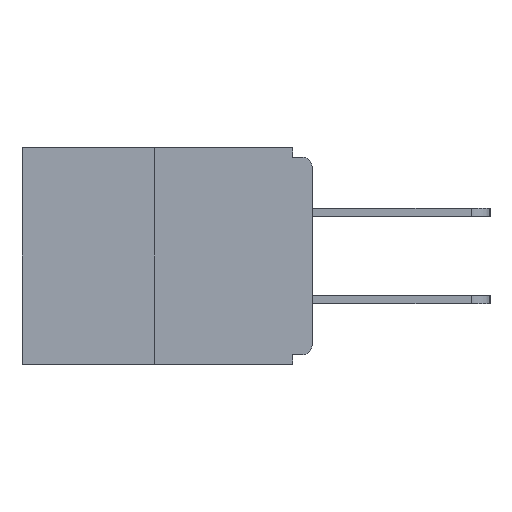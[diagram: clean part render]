
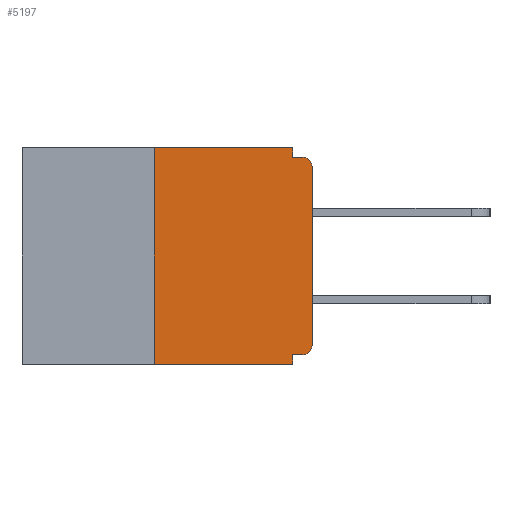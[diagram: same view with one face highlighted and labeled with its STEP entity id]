
A CAD part, left-side view. The second image highlights one B-rep face of the part: STEP entity #5197.
In plain terms, the highlighted planar face has unit normal (-1, 0, 0).
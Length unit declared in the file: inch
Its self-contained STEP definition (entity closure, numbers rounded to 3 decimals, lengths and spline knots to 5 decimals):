
#110 = PLANE ( 'NONE',  #16989 ) ;
#661 = VERTEX_POINT ( 'NONE', #16319 ) ;
#769 = EDGE_CURVE ( 'NONE', #11930, #15384, #20797, .T. ) ;
#1555 = CIRCLE ( 'NONE', #10904, 0.015 ) ;
#2557 = EDGE_CURVE ( 'NONE', #4205, #16523, #3024, .T. ) ;
#2778 = CARTESIAN_POINT ( 'NONE',  ( 0., 0.015, -0.328 ) ) ;
#2832 = CARTESIAN_POINT ( 'NONE',  ( 0., 0.031, -0.015 ) ) ;
#2899 = CARTESIAN_POINT ( 'NONE',  ( 0., 0., -0.313 ) ) ;
#3024 = LINE ( 'NONE', #4188, #15952 ) ;
#4046 = ORIENTED_EDGE ( 'NONE', *, *, #14944, .T. ) ;
#4188 = CARTESIAN_POINT ( 'NONE',  ( 0., 0.25, 0. ) ) ;
#4205 = VERTEX_POINT ( 'NONE', #7496 ) ;
#4306 = ORIENTED_EDGE ( 'NONE', *, *, #20389, .T. ) ;
#4655 = DIRECTION ( 'NONE',  ( 0., -1., 0. ) ) ;
#4814 = DIRECTION ( 'NONE',  ( -1., 0., 0. ) ) ;
#4856 = DIRECTION ( 'NONE',  ( -1., 0., 0. ) ) ;
#5109 = VERTEX_POINT ( 'NONE', #2899 ) ;
#5148 = EDGE_CURVE ( 'NONE', #15314, #5109, #1555, .T. ) ;
#5197 = ADVANCED_FACE ( 'NONE', ( #12898 ), #110, .F. ) ;
#5567 = CARTESIAN_POINT ( 'NONE',  ( 0., 0., -0.328 ) ) ;
#5944 = VECTOR ( 'NONE', #19367, 39.37008 ) ;
#6068 = VECTOR ( 'NONE', #7890, 39.37008 ) ;
#6478 = VECTOR ( 'NONE', #12403, 39.37008 ) ;
#7496 = CARTESIAN_POINT ( 'NONE',  ( 0., 0.25, -0.343 ) ) ;
#7890 = DIRECTION ( 'NONE',  ( 0., -1., 0. ) ) ;
#7942 = LINE ( 'NONE', #21148, #21616 ) ;
#7963 = LINE ( 'NONE', #11263, #16917 ) ;
#7977 = EDGE_CURVE ( 'NONE', #11602, #8048, #14386, .T. ) ;
#8048 = VERTEX_POINT ( 'NONE', #2832 ) ;
#8356 = DIRECTION ( 'NONE',  ( 0., 0., -1. ) ) ;
#8370 = EDGE_CURVE ( 'NONE', #15314, #661, #21219, .T. ) ;
#9469 = ORIENTED_EDGE ( 'NONE', *, *, #11929, .F. ) ;
#10443 = ORIENTED_EDGE ( 'NONE', *, *, #16659, .F. ) ;
#10861 = DIRECTION ( 'NONE',  ( 0., 0., 1. ) ) ;
#10904 = AXIS2_PLACEMENT_3D ( 'NONE', #11643, #4814, #8356 ) ;
#10963 = DIRECTION ( 'NONE',  ( 0., 0., -1. ) ) ;
#11066 = CARTESIAN_POINT ( 'NONE',  ( 0., 0.015, -0.015 ) ) ;
#11261 = CARTESIAN_POINT ( 'NONE',  ( 0., 0., -0.03 ) ) ;
#11263 = CARTESIAN_POINT ( 'NONE',  ( 0., 0., -0.015 ) ) ;
#11377 = ORIENTED_EDGE ( 'NONE', *, *, #2557, .F. ) ;
#11425 = AXIS2_PLACEMENT_3D ( 'NONE', #14711, #4856, #13168 ) ;
#11479 = VECTOR ( 'NONE', #17538, 39.37008 ) ;
#11602 = VERTEX_POINT ( 'NONE', #13052 ) ;
#11643 = CARTESIAN_POINT ( 'NONE',  ( 0., 0.015, -0.313 ) ) ;
#11929 = EDGE_CURVE ( 'NONE', #16523, #11602, #21688, .T. ) ;
#11930 = VERTEX_POINT ( 'NONE', #11261 ) ;
#12188 = LINE ( 'NONE', #20577, #19034 ) ;
#12294 = CARTESIAN_POINT ( 'NONE',  ( 0., 0.46, -0.343 ) ) ;
#12403 = DIRECTION ( 'NONE',  ( 0., 0., -1. ) ) ;
#12566 = ORIENTED_EDGE ( 'NONE', *, *, #20131, .F. ) ;
#12898 = FACE_OUTER_BOUND ( 'NONE', #19009, .T. ) ;
#13052 = CARTESIAN_POINT ( 'NONE',  ( 0., 0.031, 0. ) ) ;
#13168 = DIRECTION ( 'NONE',  ( 0., 0., -1. ) ) ;
#13526 = ORIENTED_EDGE ( 'NONE', *, *, #8370, .F. ) ;
#13781 = ORIENTED_EDGE ( 'NONE', *, *, #5148, .T. ) ;
#13965 = CARTESIAN_POINT ( 'NONE',  ( 0., 0.031, 0. ) ) ;
#14005 = CARTESIAN_POINT ( 'NONE',  ( 0., 0.25, 0. ) ) ;
#14386 = LINE ( 'NONE', #13965, #6478 ) ;
#14711 = CARTESIAN_POINT ( 'NONE',  ( 0., 0.015, -0.03 ) ) ;
#14944 = EDGE_CURVE ( 'NONE', #4205, #18016, #14945, .T. ) ;
#14945 = LINE ( 'NONE', #12294, #5944 ) ;
#15238 = ORIENTED_EDGE ( 'NONE', *, *, #7977, .F. ) ;
#15297 = CARTESIAN_POINT ( 'NONE',  ( 0., 0.46, 0. ) ) ;
#15314 = VERTEX_POINT ( 'NONE', #2778 ) ;
#15384 = VERTEX_POINT ( 'NONE', #11066 ) ;
#15557 = DIRECTION ( 'NONE',  ( 0., 0., 1. ) ) ;
#15952 = VECTOR ( 'NONE', #10861, 39.37008 ) ;
#16319 = CARTESIAN_POINT ( 'NONE',  ( 0., 0.031, -0.328 ) ) ;
#16523 = VERTEX_POINT ( 'NONE', #14005 ) ;
#16659 = EDGE_CURVE ( 'NONE', #661, #18016, #7942, .T. ) ;
#16917 = VECTOR ( 'NONE', #4655, 39.37008 ) ;
#16989 = AXIS2_PLACEMENT_3D ( 'NONE', #15297, #18725, #17022 ) ;
#17022 = DIRECTION ( 'NONE',  ( 0., 0., -1. ) ) ;
#17538 = DIRECTION ( 'NONE',  ( 0., 1., 0. ) ) ;
#18016 = VERTEX_POINT ( 'NONE', #19266 ) ;
#18725 = DIRECTION ( 'NONE',  ( 1., 0., 0. ) ) ;
#19009 = EDGE_LOOP ( 'NONE', ( #9469, #11377, #4046, #10443, #13526, #13781, #4306, #20323, #12566, #15238 ) ) ;
#19034 = VECTOR ( 'NONE', #15557, 39.37008 ) ;
#19266 = CARTESIAN_POINT ( 'NONE',  ( 0., 0.031, -0.343 ) ) ;
#19367 = DIRECTION ( 'NONE',  ( 0., -1., 0. ) ) ;
#20131 = EDGE_CURVE ( 'NONE', #8048, #15384, #7963, .T. ) ;
#20323 = ORIENTED_EDGE ( 'NONE', *, *, #769, .T. ) ;
#20389 = EDGE_CURVE ( 'NONE', #5109, #11930, #12188, .T. ) ;
#20577 = CARTESIAN_POINT ( 'NONE',  ( 0., 0., 0. ) ) ;
#20797 = CIRCLE ( 'NONE', #11425, 0.015 ) ;
#21148 = CARTESIAN_POINT ( 'NONE',  ( 0., 0.031, -0.343 ) ) ;
#21219 = LINE ( 'NONE', #5567, #11479 ) ;
#21519 = CARTESIAN_POINT ( 'NONE',  ( 0., 0.46, 0. ) ) ;
#21616 = VECTOR ( 'NONE', #10963, 39.37008 ) ;
#21688 = LINE ( 'NONE', #21519, #6068 ) ;
